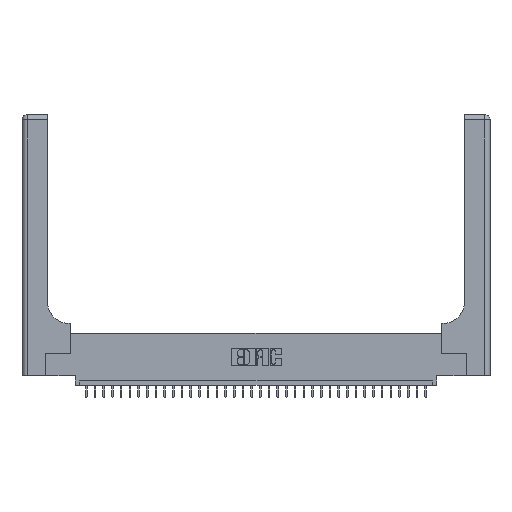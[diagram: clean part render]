
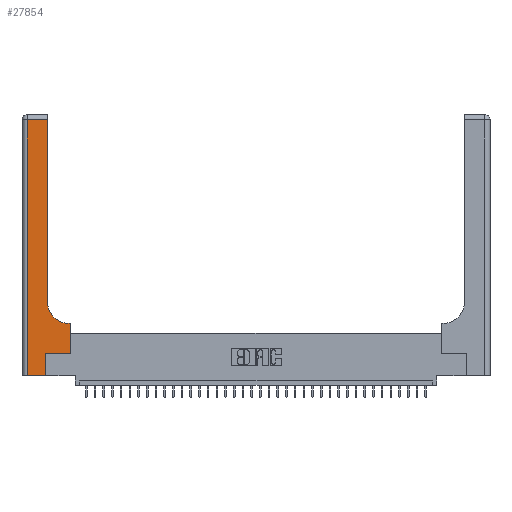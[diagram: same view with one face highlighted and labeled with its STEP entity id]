
A CAD part, top view. The second image highlights one B-rep face of the part: STEP entity #27854.
In plain terms, the highlighted planar face has unit normal (0, 0, 1).
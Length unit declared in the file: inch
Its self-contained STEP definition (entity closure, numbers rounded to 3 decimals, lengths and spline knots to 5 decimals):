
#152 = LINE ( 'NONE', #2859, #17384 ) ;
#1151 = CARTESIAN_POINT ( 'NONE',  ( 0.5415, 0.85, 0.37 ) ) ;
#2724 = EDGE_CURVE ( 'NONE', #34711, #14230, #27389, .T. ) ;
#2859 = CARTESIAN_POINT ( 'NONE',  ( 0.2915, 0.6, 0.37 ) ) ;
#3666 = LINE ( 'NONE', #20163, #26769 ) ;
#3973 = EDGE_CURVE ( 'NONE', #14230, #24829, #31289, .T. ) ;
#4122 = ORIENTED_EDGE ( 'NONE', *, *, #7138, .T. ) ;
#5439 = ORIENTED_EDGE ( 'NONE', *, *, #31482, .T. ) ;
#5928 = LINE ( 'NONE', #12104, #23215 ) ;
#6459 = DIRECTION ( 'NONE',  ( -1., 0., 0. ) ) ;
#6481 = CARTESIAN_POINT ( 'NONE',  ( 0., 2.94, 0.37 ) ) ;
#6991 = VERTEX_POINT ( 'NONE', #17855 ) ;
#7138 = EDGE_CURVE ( 'NONE', #24829, #8882, #30254, .T. ) ;
#7730 = CARTESIAN_POINT ( 'NONE',  ( 0.2915, 0.85, 0.37 ) ) ;
#7909 = CARTESIAN_POINT ( 'NONE',  ( 0.5415, 0.6, 0.37 ) ) ;
#8020 = EDGE_LOOP ( 'NONE', ( #20420, #10323, #4122, #5439, #27044, #11371, #15223, #22942, #18639 ) ) ;
#8036 = LINE ( 'NONE', #33036, #25668 ) ;
#8695 = CARTESIAN_POINT ( 'NONE',  ( 0.269, 0., 0.37 ) ) ;
#8882 = VERTEX_POINT ( 'NONE', #35136 ) ;
#9838 = CARTESIAN_POINT ( 'NONE',  ( 0.2915, 2.94, 0.37 ) ) ;
#10294 = CARTESIAN_POINT ( 'NONE',  ( 0.06, 2.94, 0.37 ) ) ;
#10323 = ORIENTED_EDGE ( 'NONE', *, *, #3973, .T. ) ;
#10381 = DIRECTION ( 'NONE',  ( 0., 1., 0. ) ) ;
#10685 = VERTEX_POINT ( 'NONE', #21503 ) ;
#11371 = ORIENTED_EDGE ( 'NONE', *, *, #32317, .T. ) ;
#11933 = DIRECTION ( 'NONE',  ( 0., 1., 0. ) ) ;
#12104 = CARTESIAN_POINT ( 'NONE',  ( 0.269, 0., 0.37 ) ) ;
#12245 = DIRECTION ( 'NONE',  ( 0., 0., -1. ) ) ;
#13395 = AXIS2_PLACEMENT_3D ( 'NONE', #17894, #15544, #6459 ) ;
#14230 = VERTEX_POINT ( 'NONE', #9838 ) ;
#14659 = LINE ( 'NONE', #28181, #19833 ) ;
#14757 = DIRECTION ( 'NONE',  ( 1., 0., 0. ) ) ;
#14932 = VECTOR ( 'NONE', #32973, 39.37008 ) ;
#15223 = ORIENTED_EDGE ( 'NONE', *, *, #24137, .T. ) ;
#15544 = DIRECTION ( 'NONE',  ( 0., 0., -1. ) ) ;
#16393 = AXIS2_PLACEMENT_3D ( 'NONE', #1151, #12245, #26131 ) ;
#16409 = DIRECTION ( 'NONE',  ( 0., 1., 0. ) ) ;
#17384 = VECTOR ( 'NONE', #27470, 39.37008 ) ;
#17570 = DIRECTION ( 'NONE',  ( -1., 0., 0. ) ) ;
#17855 = CARTESIAN_POINT ( 'NONE',  ( 0.269, 0.25, 0.37 ) ) ;
#17894 = CARTESIAN_POINT ( 'NONE',  ( 0., 3., 0.37 ) ) ;
#18540 = VECTOR ( 'NONE', #17570, 39.37008 ) ;
#18639 = ORIENTED_EDGE ( 'NONE', *, *, #22615, .T. ) ;
#18812 = EDGE_CURVE ( 'NONE', #28777, #33547, #152, .T. ) ;
#19833 = VECTOR ( 'NONE', #20245, 39.37008 ) ;
#20163 = CARTESIAN_POINT ( 'NONE',  ( 0.269, 0.25, 0.37 ) ) ;
#20245 = DIRECTION ( 'NONE',  ( 1., 0., 0. ) ) ;
#20420 = ORIENTED_EDGE ( 'NONE', *, *, #2724, .T. ) ;
#21503 = CARTESIAN_POINT ( 'NONE',  ( 0.5585, 0.25, 0.37 ) ) ;
#22615 = EDGE_CURVE ( 'NONE', #33547, #34711, #35414, .T. ) ;
#22942 = ORIENTED_EDGE ( 'NONE', *, *, #18812, .T. ) ;
#23104 = PLANE ( 'NONE',  #13395 ) ;
#23215 = VECTOR ( 'NONE', #11933, 39.37008 ) ;
#24137 = EDGE_CURVE ( 'NONE', #10685, #28777, #8036, .T. ) ;
#24829 = VERTEX_POINT ( 'NONE', #10294 ) ;
#25668 = VECTOR ( 'NONE', #16409, 39.37008 ) ;
#26131 = DIRECTION ( 'NONE',  ( 1., 0., 0. ) ) ;
#26769 = VECTOR ( 'NONE', #14757, 39.37008 ) ;
#27044 = ORIENTED_EDGE ( 'NONE', *, *, #30277, .T. ) ;
#27389 = LINE ( 'NONE', #35181, #30525 ) ;
#27470 = DIRECTION ( 'NONE',  ( -1., 0., 0. ) ) ;
#27854 = ADVANCED_FACE ( 'NONE', ( #31266 ), #23104, .F. ) ;
#28181 = CARTESIAN_POINT ( 'NONE',  ( 0., 0., 0.37 ) ) ;
#28777 = VERTEX_POINT ( 'NONE', #35449 ) ;
#29820 = VERTEX_POINT ( 'NONE', #8695 ) ;
#30254 = LINE ( 'NONE', #32606, #14932 ) ;
#30277 = EDGE_CURVE ( 'NONE', #29820, #6991, #5928, .T. ) ;
#30525 = VECTOR ( 'NONE', #10381, 39.37008 ) ;
#31266 = FACE_OUTER_BOUND ( 'NONE', #8020, .T. ) ;
#31289 = LINE ( 'NONE', #6481, #18540 ) ;
#31482 = EDGE_CURVE ( 'NONE', #8882, #29820, #14659, .T. ) ;
#32317 = EDGE_CURVE ( 'NONE', #6991, #10685, #3666, .T. ) ;
#32606 = CARTESIAN_POINT ( 'NONE',  ( 0.06, 3., 0.37 ) ) ;
#32973 = DIRECTION ( 'NONE',  ( 0., -1., 0. ) ) ;
#33036 = CARTESIAN_POINT ( 'NONE',  ( 0.5585, 0.25, 0.37 ) ) ;
#33547 = VERTEX_POINT ( 'NONE', #7909 ) ;
#34711 = VERTEX_POINT ( 'NONE', #7730 ) ;
#35136 = CARTESIAN_POINT ( 'NONE',  ( 0.06, 0., 0.37 ) ) ;
#35181 = CARTESIAN_POINT ( 'NONE',  ( 0.2915, 3., 0.37 ) ) ;
#35414 = CIRCLE ( 'NONE', #16393, 0.25 ) ;
#35449 = CARTESIAN_POINT ( 'NONE',  ( 0.5585, 0.6, 0.37 ) ) ;
